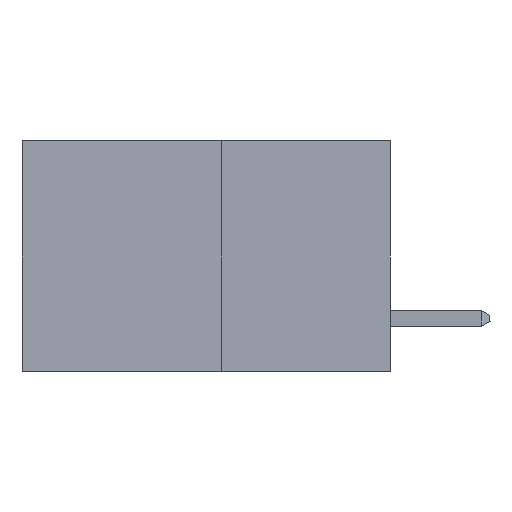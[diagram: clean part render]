
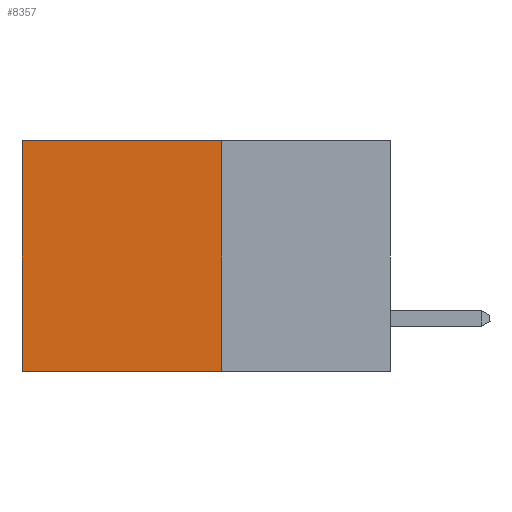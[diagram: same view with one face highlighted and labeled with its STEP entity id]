
A CAD part, left-side view. The second image highlights one B-rep face of the part: STEP entity #8357.
In plain terms, the highlighted planar face has unit normal (-1, 0, 0).
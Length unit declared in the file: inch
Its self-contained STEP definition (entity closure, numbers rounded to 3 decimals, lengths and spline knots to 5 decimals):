
#7 = LINE ( 'NONE', #11274, #9114 ) ;
#106 = CARTESIAN_POINT ( 'NONE',  ( 0.277, 0.59, 0. ) ) ;
#509 = EDGE_CURVE ( 'NONE', #10467, #2924, #1186, .T. ) ;
#588 = CARTESIAN_POINT ( 'NONE',  ( 0.277, 0.27, 0. ) ) ;
#645 = LINE ( 'NONE', #7492, #2889 ) ;
#1186 = LINE ( 'NONE', #11318, #6386 ) ;
#1467 = ORIENTED_EDGE ( 'NONE', *, *, #9729, .F. ) ;
#1913 = ORIENTED_EDGE ( 'NONE', *, *, #3396, .T. ) ;
#2030 = AXIS2_PLACEMENT_3D ( 'NONE', #9191, #8908, #9556 ) ;
#2889 = VECTOR ( 'NONE', #5490, 39.37008 ) ;
#2924 = VERTEX_POINT ( 'NONE', #10334 ) ;
#2937 = EDGE_CURVE ( 'NONE', #10467, #7623, #5902, .T. ) ;
#3396 = EDGE_CURVE ( 'NONE', #7623, #5530, #645, .T. ) ;
#3398 = DIRECTION ( 'NONE',  ( 0., 1., 0. ) ) ;
#5490 = DIRECTION ( 'NONE',  ( 0., 0., -1. ) ) ;
#5530 = VERTEX_POINT ( 'NONE', #6393 ) ;
#5699 = EDGE_LOOP ( 'NONE', ( #1913, #1467, #6554, #5814 ) ) ;
#5814 = ORIENTED_EDGE ( 'NONE', *, *, #2937, .T. ) ;
#5902 = LINE ( 'NONE', #588, #8510 ) ;
#6386 = VECTOR ( 'NONE', #7518, 39.37008 ) ;
#6393 = CARTESIAN_POINT ( 'NONE',  ( 0.277, 0.59, -0.37 ) ) ;
#6554 = ORIENTED_EDGE ( 'NONE', *, *, #509, .F. ) ;
#7181 = CARTESIAN_POINT ( 'NONE',  ( 0.277, 0.27, 0. ) ) ;
#7492 = CARTESIAN_POINT ( 'NONE',  ( 0.277, 0.59, -0.37 ) ) ;
#7518 = DIRECTION ( 'NONE',  ( 0., 0., -1. ) ) ;
#7623 = VERTEX_POINT ( 'NONE', #106 ) ;
#8357 = ADVANCED_FACE ( 'NONE', ( #9291 ), #9153, .F. ) ;
#8510 = VECTOR ( 'NONE', #9095, 39.37008 ) ;
#8908 = DIRECTION ( 'NONE',  ( 1., 0., 0. ) ) ;
#9095 = DIRECTION ( 'NONE',  ( 0., 1., 0. ) ) ;
#9114 = VECTOR ( 'NONE', #3398, 39.37008 ) ;
#9153 = PLANE ( 'NONE',  #2030 ) ;
#9191 = CARTESIAN_POINT ( 'NONE',  ( 0.277, 0.27, -0.37 ) ) ;
#9291 = FACE_OUTER_BOUND ( 'NONE', #5699, .T. ) ;
#9556 = DIRECTION ( 'NONE',  ( 0., 0., -1. ) ) ;
#9729 = EDGE_CURVE ( 'NONE', #2924, #5530, #7, .T. ) ;
#10334 = CARTESIAN_POINT ( 'NONE',  ( 0.277, 0.27, -0.37 ) ) ;
#10467 = VERTEX_POINT ( 'NONE', #7181 ) ;
#11274 = CARTESIAN_POINT ( 'NONE',  ( 0.277, 0.27, -0.37 ) ) ;
#11318 = CARTESIAN_POINT ( 'NONE',  ( 0.277, 0.27, -0.37 ) ) ;
